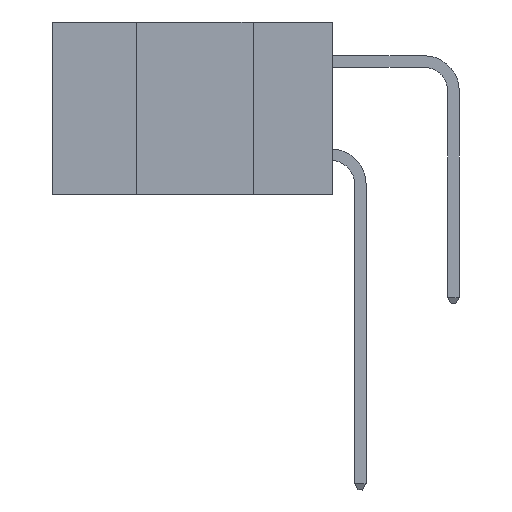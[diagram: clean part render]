
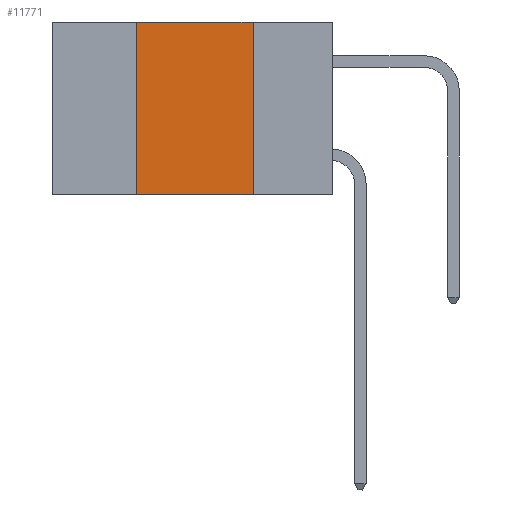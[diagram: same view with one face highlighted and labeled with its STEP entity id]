
A CAD part, left-side view. The second image highlights one B-rep face of the part: STEP entity #11771.
In plain terms, the highlighted planar face has unit normal (-1, 0, 0).
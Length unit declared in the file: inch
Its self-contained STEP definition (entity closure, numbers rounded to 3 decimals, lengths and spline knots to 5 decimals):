
#126 = ORIENTED_EDGE ( 'NONE', *, *, #10351, .F. ) ;
#820 = AXIS2_PLACEMENT_3D ( 'NONE', #19935, #9685, #21583 ) ;
#2076 = CARTESIAN_POINT ( 'NONE',  ( 0., 0.17, -0.37 ) ) ;
#3071 = CARTESIAN_POINT ( 'NONE',  ( 0., 0.6, 0. ) ) ;
#3169 = PLANE ( 'NONE',  #820 ) ;
#3557 = DIRECTION ( 'NONE',  ( 0., -1., 0. ) ) ;
#3679 = DIRECTION ( 'NONE',  ( 0., 0., -1. ) ) ;
#5355 = LINE ( 'NONE', #18822, #9469 ) ;
#5805 = DIRECTION ( 'NONE',  ( 0., 0., 1. ) ) ;
#6027 = CARTESIAN_POINT ( 'NONE',  ( 0., 0.42, -0.37 ) ) ;
#7110 = VERTEX_POINT ( 'NONE', #12293 ) ;
#8083 = ORIENTED_EDGE ( 'NONE', *, *, #12456, .T. ) ;
#9469 = VECTOR ( 'NONE', #3679, 39.37008 ) ;
#9685 = DIRECTION ( 'NONE',  ( 1., 0., 0. ) ) ;
#10351 = EDGE_CURVE ( 'NONE', #7110, #19590, #18193, .T. ) ;
#10624 = EDGE_CURVE ( 'NONE', #15693, #7110, #14204, .T. ) ;
#11771 = ADVANCED_FACE ( 'NONE', ( #19732 ), #3169, .F. ) ;
#12293 = CARTESIAN_POINT ( 'NONE',  ( 0., 0.42, 0. ) ) ;
#12328 = CARTESIAN_POINT ( 'NONE',  ( 0., 0.17, 0. ) ) ;
#12456 = EDGE_CURVE ( 'NONE', #15693, #18942, #18689, .T. ) ;
#12604 = EDGE_LOOP ( 'NONE', ( #18594, #126, #12755, #8083 ) ) ;
#12700 = DIRECTION ( 'NONE',  ( 0., -1., 0. ) ) ;
#12755 = ORIENTED_EDGE ( 'NONE', *, *, #10624, .F. ) ;
#13256 = VECTOR ( 'NONE', #3557, 39.37008 ) ;
#13780 = CARTESIAN_POINT ( 'NONE',  ( 0., 0.42, -0.37 ) ) ;
#13986 = VECTOR ( 'NONE', #12700, 39.37008 ) ;
#14204 = LINE ( 'NONE', #13780, #21044 ) ;
#15494 = CARTESIAN_POINT ( 'NONE',  ( 0., 0.6, -0.37 ) ) ;
#15693 = VERTEX_POINT ( 'NONE', #6027 ) ;
#16435 = EDGE_CURVE ( 'NONE', #19590, #18942, #5355, .T. ) ;
#18193 = LINE ( 'NONE', #3071, #13986 ) ;
#18594 = ORIENTED_EDGE ( 'NONE', *, *, #16435, .F. ) ;
#18689 = LINE ( 'NONE', #15494, #13256 ) ;
#18822 = CARTESIAN_POINT ( 'NONE',  ( 0., 0.17, -0.37 ) ) ;
#18942 = VERTEX_POINT ( 'NONE', #2076 ) ;
#19590 = VERTEX_POINT ( 'NONE', #12328 ) ;
#19732 = FACE_OUTER_BOUND ( 'NONE', #12604, .T. ) ;
#19935 = CARTESIAN_POINT ( 'NONE',  ( 0., 0.6, 0. ) ) ;
#21044 = VECTOR ( 'NONE', #5805, 39.37008 ) ;
#21583 = DIRECTION ( 'NONE',  ( 0., 0., -1. ) ) ;
